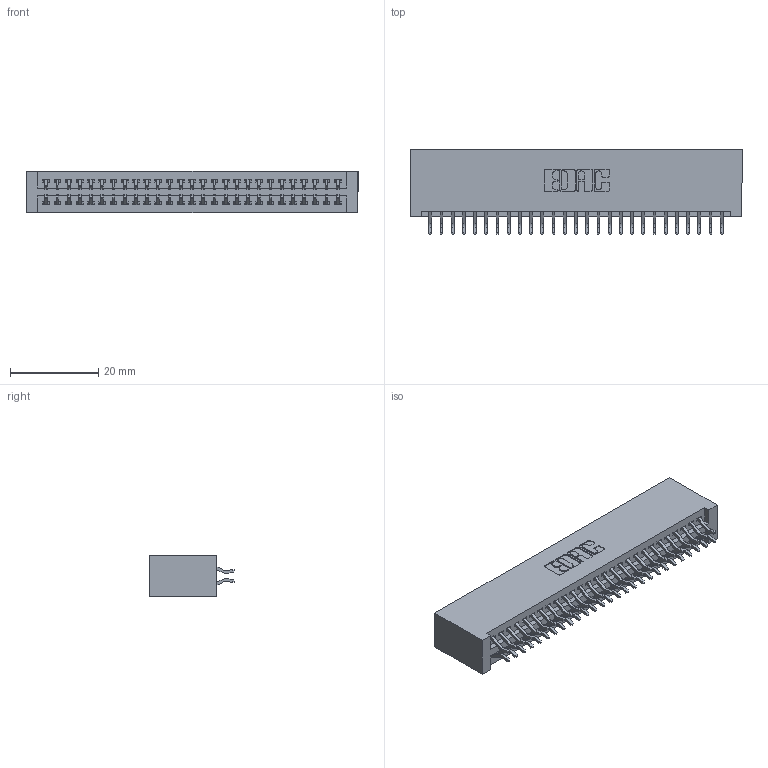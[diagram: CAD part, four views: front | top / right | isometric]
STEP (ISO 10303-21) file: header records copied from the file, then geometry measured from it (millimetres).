
FILE_DESCRIPTION (( 'STEP AP203' ), '1' );
FILE_NAME ('395-054-556-201.STEP', '2018-11-21T11:27:46', ( '' ), ( '' ), 'SwSTEP 2.0', 'SolidWorks 2016', '' );
FILE_SCHEMA (( 'CONFIG_CONTROL_DESIGN' ));
Length unit declared in the file: inch
Products named in the file (3): 345 Part_No Mounting Lugs; 395-054-556-201; 345-292-001_556 Tail
Assembly tree (55 placements, depth 2):
  395-054-556-201
    345 Part_No Mounting Lugs
    345-292-001_556 Tail  x54
Bounding box: 75.18 x 19.24 x 9.4 mm (x, y, z)
Volume: 7778 mm3; surface area: 11462.7 mm2
Topology: 55 solids, 55 shells, 3142 faces, 9335 edges, 6150 vertices
Faces by surface type: plane 2074, cylinder 1068
Entity records: 23147 total; most frequent: CARTESIAN_POINT 3908, ORIENTED_EDGE 3830, DIRECTION 3447, EDGE_CURVE 1915, LINE 1675, VECTOR 1675, VERTEX_POINT 1274, AXIS2_PLACEMENT_3D 886
